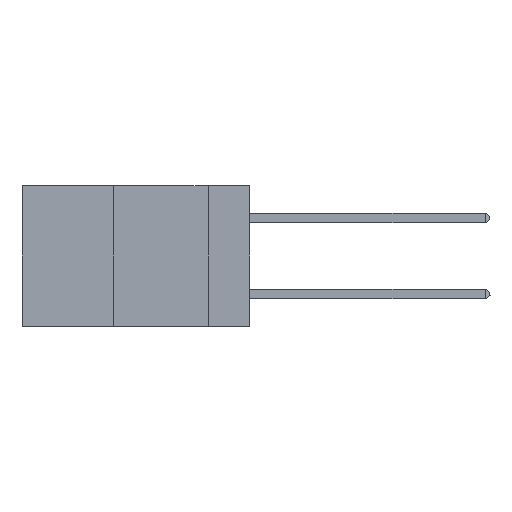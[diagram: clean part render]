
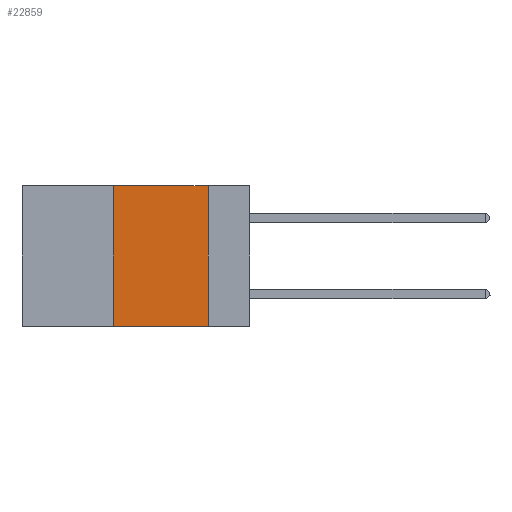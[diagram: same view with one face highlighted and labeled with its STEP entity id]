
A CAD part, left-side view. The second image highlights one B-rep face of the part: STEP entity #22859.
In plain terms, the highlighted planar face has unit normal (-1, 0, 0).
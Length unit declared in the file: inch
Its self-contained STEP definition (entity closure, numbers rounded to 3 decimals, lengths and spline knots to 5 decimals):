
#364 = EDGE_CURVE ( 'NONE', #14801, #8852, #10839, .T. ) ;
#788 = ORIENTED_EDGE ( 'NONE', *, *, #364, .T. ) ;
#2219 = VECTOR ( 'NONE', #15475, 39.37008 ) ;
#2380 = EDGE_CURVE ( 'NONE', #14801, #17393, #12948, .T. ) ;
#2872 = DIRECTION ( 'NONE',  ( 0., 0., -1. ) ) ;
#4720 = AXIS2_PLACEMENT_3D ( 'NONE', #12873, #18922, #2872 ) ;
#4731 = CARTESIAN_POINT ( 'NONE',  ( 0., 0.36, 0. ) ) ;
#4786 = VERTEX_POINT ( 'NONE', #13351 ) ;
#5360 = EDGE_CURVE ( 'NONE', #17393, #4786, #13106, .T. ) ;
#5545 = ORIENTED_EDGE ( 'NONE', *, *, #2380, .F. ) ;
#7471 = CARTESIAN_POINT ( 'NONE',  ( 0., 0.36, -0.37 ) ) ;
#8335 = LINE ( 'NONE', #13100, #13716 ) ;
#8701 = CARTESIAN_POINT ( 'NONE',  ( 0., 0.6, -0.37 ) ) ;
#8852 = VERTEX_POINT ( 'NONE', #19023 ) ;
#8986 = PLANE ( 'NONE',  #4720 ) ;
#9086 = CARTESIAN_POINT ( 'NONE',  ( 0., 0.36, 0. ) ) ;
#10206 = DIRECTION ( 'NONE',  ( 0., -1., 0. ) ) ;
#10839 = LINE ( 'NONE', #8701, #14033 ) ;
#11210 = FACE_OUTER_BOUND ( 'NONE', #13552, .T. ) ;
#12873 = CARTESIAN_POINT ( 'NONE',  ( 0., 0.6, 0. ) ) ;
#12948 = LINE ( 'NONE', #4731, #2219 ) ;
#13100 = CARTESIAN_POINT ( 'NONE',  ( 0., 0.11, 0. ) ) ;
#13106 = LINE ( 'NONE', #24539, #14990 ) ;
#13351 = CARTESIAN_POINT ( 'NONE',  ( 0., 0.11, 0. ) ) ;
#13552 = EDGE_LOOP ( 'NONE', ( #22767, #18706, #5545, #788 ) ) ;
#13716 = VECTOR ( 'NONE', #15187, 39.37008 ) ;
#14033 = VECTOR ( 'NONE', #20728, 39.37008 ) ;
#14801 = VERTEX_POINT ( 'NONE', #7471 ) ;
#14990 = VECTOR ( 'NONE', #10206, 39.37008 ) ;
#15187 = DIRECTION ( 'NONE',  ( 0., 0., -1. ) ) ;
#15475 = DIRECTION ( 'NONE',  ( 0., 0., 1. ) ) ;
#17393 = VERTEX_POINT ( 'NONE', #9086 ) ;
#18706 = ORIENTED_EDGE ( 'NONE', *, *, #5360, .F. ) ;
#18922 = DIRECTION ( 'NONE',  ( 1., 0., 0. ) ) ;
#19023 = CARTESIAN_POINT ( 'NONE',  ( 0., 0.11, -0.37 ) ) ;
#20728 = DIRECTION ( 'NONE',  ( 0., -1., 0. ) ) ;
#22767 = ORIENTED_EDGE ( 'NONE', *, *, #24739, .F. ) ;
#22859 = ADVANCED_FACE ( 'NONE', ( #11210 ), #8986, .F. ) ;
#24539 = CARTESIAN_POINT ( 'NONE',  ( 0., 0.6, 0. ) ) ;
#24739 = EDGE_CURVE ( 'NONE', #4786, #8852, #8335, .T. ) ;
